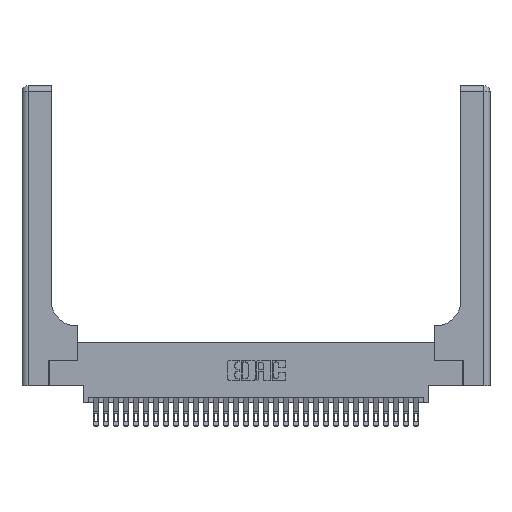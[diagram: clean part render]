
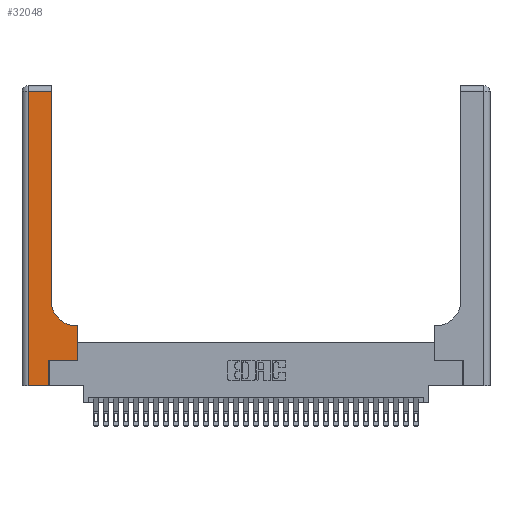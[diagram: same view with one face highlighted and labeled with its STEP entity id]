
A CAD part, top view. The second image highlights one B-rep face of the part: STEP entity #32048.
In plain terms, the highlighted planar face has unit normal (0, 0, 1).
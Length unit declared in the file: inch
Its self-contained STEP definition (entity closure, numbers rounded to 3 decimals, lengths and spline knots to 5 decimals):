
#95 = EDGE_LOOP ( 'NONE', ( #4274, #25356, #12806, #21076, #8277, #18378, #31565, #19498, #27650 ) ) ;
#706 = VERTEX_POINT ( 'NONE', #17264 ) ;
#941 = EDGE_CURVE ( 'NONE', #10120, #706, #10653, .T. ) ;
#1394 = VERTEX_POINT ( 'NONE', #9827 ) ;
#1470 = VERTEX_POINT ( 'NONE', #6524 ) ;
#1474 = VERTEX_POINT ( 'NONE', #6416 ) ;
#1535 = VECTOR ( 'NONE', #3155, 39.37008 ) ;
#1546 = EDGE_CURVE ( 'NONE', #706, #4720, #15094, .T. ) ;
#2293 = CARTESIAN_POINT ( 'NONE',  ( 0.269, 0., 0.37 ) ) ;
#3073 = CARTESIAN_POINT ( 'NONE',  ( 0., 3., 0.37 ) ) ;
#3154 = LINE ( 'NONE', #21030, #1535 ) ;
#3155 = DIRECTION ( 'NONE',  ( 1., 0., 0. ) ) ;
#3438 = DIRECTION ( 'NONE',  ( -1., 0., 0. ) ) ;
#3624 = CARTESIAN_POINT ( 'NONE',  ( 0., 0., 0.37 ) ) ;
#3791 = CARTESIAN_POINT ( 'NONE',  ( 0., 2.94, 0.37 ) ) ;
#4165 = DIRECTION ( 'NONE',  ( 0., 0., -1. ) ) ;
#4274 = ORIENTED_EDGE ( 'NONE', *, *, #941, .T. ) ;
#4597 = VECTOR ( 'NONE', #12063, 39.37008 ) ;
#4720 = VERTEX_POINT ( 'NONE', #10591 ) ;
#5509 = DIRECTION ( 'NONE',  ( 0., 1., 0. ) ) ;
#5681 = CARTESIAN_POINT ( 'NONE',  ( 0.269, 0.25, 0.37 ) ) ;
#6245 = DIRECTION ( 'NONE',  ( 0., 1., 0. ) ) ;
#6416 = CARTESIAN_POINT ( 'NONE',  ( 0.5415, 0.6, 0.37 ) ) ;
#6524 = CARTESIAN_POINT ( 'NONE',  ( 0.06, 0., 0.37 ) ) ;
#6615 = LINE ( 'NONE', #23760, #32660 ) ;
#8277 = ORIENTED_EDGE ( 'NONE', *, *, #9375, .T. ) ;
#8960 = EDGE_CURVE ( 'NONE', #1470, #9180, #29175, .T. ) ;
#9180 = VERTEX_POINT ( 'NONE', #2293 ) ;
#9375 = EDGE_CURVE ( 'NONE', #9180, #10087, #11491, .T. ) ;
#9827 = CARTESIAN_POINT ( 'NONE',  ( 0.5585, 0.6, 0.37 ) ) ;
#10087 = VERTEX_POINT ( 'NONE', #5681 ) ;
#10120 = VERTEX_POINT ( 'NONE', #28584 ) ;
#10591 = CARTESIAN_POINT ( 'NONE',  ( 0.06, 2.94, 0.37 ) ) ;
#10653 = LINE ( 'NONE', #27363, #29921 ) ;
#10961 = DIRECTION ( 'NONE',  ( 0., 0., -1. ) ) ;
#11382 = CARTESIAN_POINT ( 'NONE',  ( 0.5585, 0.25, 0.37 ) ) ;
#11491 = LINE ( 'NONE', #20833, #30709 ) ;
#12063 = DIRECTION ( 'NONE',  ( 0., -1., 0. ) ) ;
#12806 = ORIENTED_EDGE ( 'NONE', *, *, #31014, .T. ) ;
#15094 = LINE ( 'NONE', #3791, #20956 ) ;
#15563 = VERTEX_POINT ( 'NONE', #16013 ) ;
#15919 = AXIS2_PLACEMENT_3D ( 'NONE', #3073, #10961, #28538 ) ;
#15968 = VECTOR ( 'NONE', #26475, 39.37008 ) ;
#16013 = CARTESIAN_POINT ( 'NONE',  ( 0.5585, 0.25, 0.37 ) ) ;
#17094 = LINE ( 'NONE', #11382, #28746 ) ;
#17264 = CARTESIAN_POINT ( 'NONE',  ( 0.2915, 2.94, 0.37 ) ) ;
#17459 = AXIS2_PLACEMENT_3D ( 'NONE', #19541, #4165, #22025 ) ;
#17684 = FACE_OUTER_BOUND ( 'NONE', #95, .T. ) ;
#18378 = ORIENTED_EDGE ( 'NONE', *, *, #32581, .T. ) ;
#18979 = DIRECTION ( 'NONE',  ( -1., 0., 0. ) ) ;
#19388 = EDGE_CURVE ( 'NONE', #1474, #10120, #28134, .T. ) ;
#19498 = ORIENTED_EDGE ( 'NONE', *, *, #30315, .T. ) ;
#19541 = CARTESIAN_POINT ( 'NONE',  ( 0.5415, 0.85, 0.37 ) ) ;
#20833 = CARTESIAN_POINT ( 'NONE',  ( 0.269, 0., 0.37 ) ) ;
#20956 = VECTOR ( 'NONE', #3438, 39.37008 ) ;
#21030 = CARTESIAN_POINT ( 'NONE',  ( 0.269, 0.25, 0.37 ) ) ;
#21076 = ORIENTED_EDGE ( 'NONE', *, *, #8960, .T. ) ;
#22025 = DIRECTION ( 'NONE',  ( 1., 0., 0. ) ) ;
#23760 = CARTESIAN_POINT ( 'NONE',  ( 0.2915, 0.6, 0.37 ) ) ;
#24609 = CARTESIAN_POINT ( 'NONE',  ( 0.06, 3., 0.37 ) ) ;
#24869 = LINE ( 'NONE', #24609, #4597 ) ;
#25356 = ORIENTED_EDGE ( 'NONE', *, *, #1546, .T. ) ;
#26041 = PLANE ( 'NONE',  #15919 ) ;
#26475 = DIRECTION ( 'NONE',  ( 1., 0., 0. ) ) ;
#27044 = DIRECTION ( 'NONE',  ( 0., 1., 0. ) ) ;
#27363 = CARTESIAN_POINT ( 'NONE',  ( 0.2915, 3., 0.37 ) ) ;
#27650 = ORIENTED_EDGE ( 'NONE', *, *, #19388, .T. ) ;
#28134 = CIRCLE ( 'NONE', #17459, 0.25 ) ;
#28538 = DIRECTION ( 'NONE',  ( -1., 0., 0. ) ) ;
#28584 = CARTESIAN_POINT ( 'NONE',  ( 0.2915, 0.85, 0.37 ) ) ;
#28746 = VECTOR ( 'NONE', #6245, 39.37008 ) ;
#29175 = LINE ( 'NONE', #3624, #15968 ) ;
#29921 = VECTOR ( 'NONE', #27044, 39.37008 ) ;
#30315 = EDGE_CURVE ( 'NONE', #1394, #1474, #6615, .T. ) ;
#30709 = VECTOR ( 'NONE', #5509, 39.37008 ) ;
#30875 = EDGE_CURVE ( 'NONE', #15563, #1394, #17094, .T. ) ;
#31014 = EDGE_CURVE ( 'NONE', #4720, #1470, #24869, .T. ) ;
#31565 = ORIENTED_EDGE ( 'NONE', *, *, #30875, .T. ) ;
#32048 = ADVANCED_FACE ( 'NONE', ( #17684 ), #26041, .F. ) ;
#32581 = EDGE_CURVE ( 'NONE', #10087, #15563, #3154, .T. ) ;
#32660 = VECTOR ( 'NONE', #18979, 39.37008 ) ;
